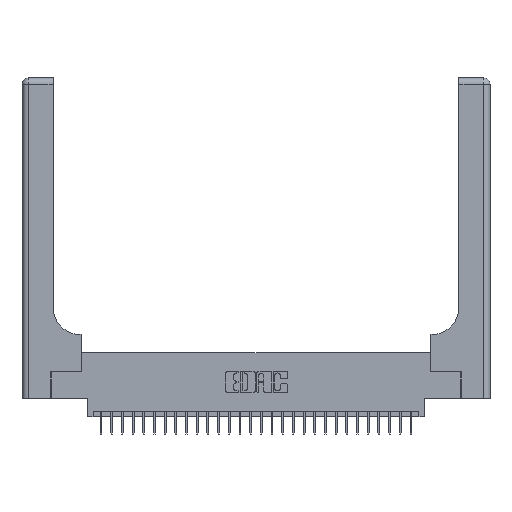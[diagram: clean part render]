
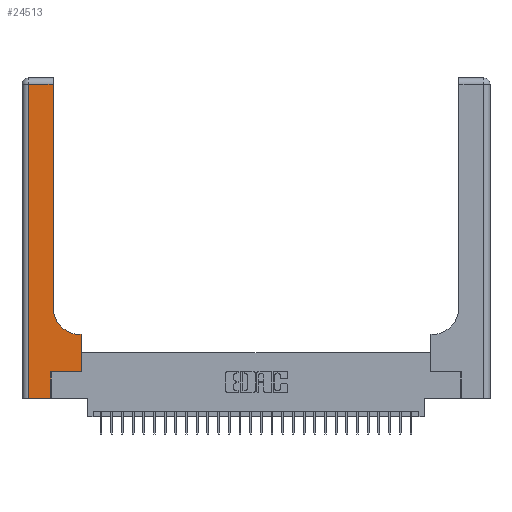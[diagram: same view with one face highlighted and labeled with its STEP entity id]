
A CAD part, top view. The second image highlights one B-rep face of the part: STEP entity #24513.
In plain terms, the highlighted planar face has unit normal (0, 0, 1).
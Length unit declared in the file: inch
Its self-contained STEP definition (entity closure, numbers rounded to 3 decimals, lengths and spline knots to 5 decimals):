
#208 = LINE ( 'NONE', #25083, #29374 ) ;
#535 = EDGE_CURVE ( 'NONE', #27362, #23395, #24442, .T. ) ;
#662 = CARTESIAN_POINT ( 'NONE',  ( 0.06, 0., 0.37 ) ) ;
#1148 = DIRECTION ( 'NONE',  ( -1., 0., 0. ) ) ;
#2259 = LINE ( 'NONE', #26321, #26646 ) ;
#2284 = CARTESIAN_POINT ( 'NONE',  ( 0.2915, 0.85, 0.37 ) ) ;
#3697 = CARTESIAN_POINT ( 'NONE',  ( 0., 2.94, 0.37 ) ) ;
#3824 = PLANE ( 'NONE',  #4101 ) ;
#3852 = DIRECTION ( 'NONE',  ( 0., 1., 0. ) ) ;
#4101 = AXIS2_PLACEMENT_3D ( 'NONE', #20369, #6271, #22706 ) ;
#4291 = ORIENTED_EDGE ( 'NONE', *, *, #8237, .T. ) ;
#4980 = ORIENTED_EDGE ( 'NONE', *, *, #15160, .T. ) ;
#5125 = FACE_OUTER_BOUND ( 'NONE', #23627, .T. ) ;
#5254 = VECTOR ( 'NONE', #14849, 39.37008 ) ;
#5312 = DIRECTION ( 'NONE',  ( 0., 1., 0. ) ) ;
#5716 = VECTOR ( 'NONE', #1148, 39.37008 ) ;
#6271 = DIRECTION ( 'NONE',  ( 0., 0., -1. ) ) ;
#6360 = EDGE_CURVE ( 'NONE', #22766, #22967, #21924, .T. ) ;
#6653 = CARTESIAN_POINT ( 'NONE',  ( 0.269, 0., 0.37 ) ) ;
#6666 = ORIENTED_EDGE ( 'NONE', *, *, #8157, .T. ) ;
#7015 = CARTESIAN_POINT ( 'NONE',  ( 0.269, 0.25, 0.37 ) ) ;
#8157 = EDGE_CURVE ( 'NONE', #9839, #30111, #13149, .T. ) ;
#8189 = ORIENTED_EDGE ( 'NONE', *, *, #9617, .T. ) ;
#8237 = EDGE_CURVE ( 'NONE', #16552, #22766, #17084, .T. ) ;
#8983 = VERTEX_POINT ( 'NONE', #662 ) ;
#9401 = CARTESIAN_POINT ( 'NONE',  ( 0.06, 3., 0.37 ) ) ;
#9480 = ORIENTED_EDGE ( 'NONE', *, *, #21877, .T. ) ;
#9617 = EDGE_CURVE ( 'NONE', #22967, #27362, #208, .T. ) ;
#9839 = VERTEX_POINT ( 'NONE', #7015 ) ;
#10365 = CARTESIAN_POINT ( 'NONE',  ( 0.2915, 2.94, 0.37 ) ) ;
#10561 = VERTEX_POINT ( 'NONE', #6653 ) ;
#10809 = CARTESIAN_POINT ( 'NONE',  ( 0.269, 0., 0.37 ) ) ;
#11026 = ORIENTED_EDGE ( 'NONE', *, *, #6360, .T. ) ;
#11726 = LINE ( 'NONE', #9401, #23301 ) ;
#11838 = DIRECTION ( 'NONE',  ( 0., -1., 0. ) ) ;
#12219 = CARTESIAN_POINT ( 'NONE',  ( 0.269, 0.25, 0.37 ) ) ;
#12527 = CARTESIAN_POINT ( 'NONE',  ( 0.2915, 0.6, 0.37 ) ) ;
#12961 = CARTESIAN_POINT ( 'NONE',  ( 0.5585, 0.25, 0.37 ) ) ;
#13076 = DIRECTION ( 'NONE',  ( 1., 0., 0. ) ) ;
#13149 = LINE ( 'NONE', #12219, #14586 ) ;
#13204 = VECTOR ( 'NONE', #13076, 39.37008 ) ;
#13293 = DIRECTION ( 'NONE',  ( 0., 0., -1. ) ) ;
#13521 = CARTESIAN_POINT ( 'NONE',  ( 0.5415, 0.6, 0.37 ) ) ;
#13581 = CARTESIAN_POINT ( 'NONE',  ( 0.06, 2.94, 0.37 ) ) ;
#14463 = CARTESIAN_POINT ( 'NONE',  ( 0.5415, 0.85, 0.37 ) ) ;
#14586 = VECTOR ( 'NONE', #21506, 39.37008 ) ;
#14849 = DIRECTION ( 'NONE',  ( -1., 0., 0. ) ) ;
#15160 = EDGE_CURVE ( 'NONE', #8983, #10561, #19318, .T. ) ;
#15926 = ORIENTED_EDGE ( 'NONE', *, *, #27289, .T. ) ;
#16552 = VERTEX_POINT ( 'NONE', #20813 ) ;
#16763 = DIRECTION ( 'NONE',  ( 1., 0., 0. ) ) ;
#17084 = LINE ( 'NONE', #12527, #5254 ) ;
#17659 = EDGE_CURVE ( 'NONE', #10561, #9839, #25005, .T. ) ;
#17689 = CARTESIAN_POINT ( 'NONE',  ( 0., 0., 0.37 ) ) ;
#19318 = LINE ( 'NONE', #17689, #13204 ) ;
#20310 = ORIENTED_EDGE ( 'NONE', *, *, #17659, .T. ) ;
#20369 = CARTESIAN_POINT ( 'NONE',  ( 0., 3., 0.37 ) ) ;
#20813 = CARTESIAN_POINT ( 'NONE',  ( 0.5585, 0.6, 0.37 ) ) ;
#21506 = DIRECTION ( 'NONE',  ( 1., 0., 0. ) ) ;
#21877 = EDGE_CURVE ( 'NONE', #23395, #8983, #11726, .T. ) ;
#21924 = CIRCLE ( 'NONE', #25441, 0.25 ) ;
#22706 = DIRECTION ( 'NONE',  ( -1., 0., 0. ) ) ;
#22766 = VERTEX_POINT ( 'NONE', #13521 ) ;
#22967 = VERTEX_POINT ( 'NONE', #2284 ) ;
#23301 = VECTOR ( 'NONE', #11838, 39.37008 ) ;
#23395 = VERTEX_POINT ( 'NONE', #13581 ) ;
#23627 = EDGE_LOOP ( 'NONE', ( #8189, #24624, #9480, #4980, #20310, #6666, #15926, #4291, #11026 ) ) ;
#24442 = LINE ( 'NONE', #3697, #5716 ) ;
#24513 = ADVANCED_FACE ( 'NONE', ( #5125 ), #3824, .F. ) ;
#24624 = ORIENTED_EDGE ( 'NONE', *, *, #535, .T. ) ;
#25005 = LINE ( 'NONE', #10809, #30392 ) ;
#25083 = CARTESIAN_POINT ( 'NONE',  ( 0.2915, 3., 0.37 ) ) ;
#25441 = AXIS2_PLACEMENT_3D ( 'NONE', #14463, #13293, #16763 ) ;
#26321 = CARTESIAN_POINT ( 'NONE',  ( 0.5585, 0.25, 0.37 ) ) ;
#26646 = VECTOR ( 'NONE', #5312, 39.37008 ) ;
#27289 = EDGE_CURVE ( 'NONE', #30111, #16552, #2259, .T. ) ;
#27362 = VERTEX_POINT ( 'NONE', #10365 ) ;
#29334 = DIRECTION ( 'NONE',  ( 0., 1., 0. ) ) ;
#29374 = VECTOR ( 'NONE', #3852, 39.37008 ) ;
#30111 = VERTEX_POINT ( 'NONE', #12961 ) ;
#30392 = VECTOR ( 'NONE', #29334, 39.37008 ) ;
